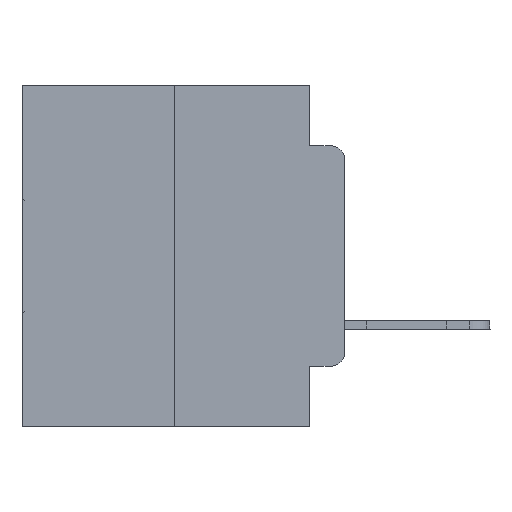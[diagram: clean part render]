
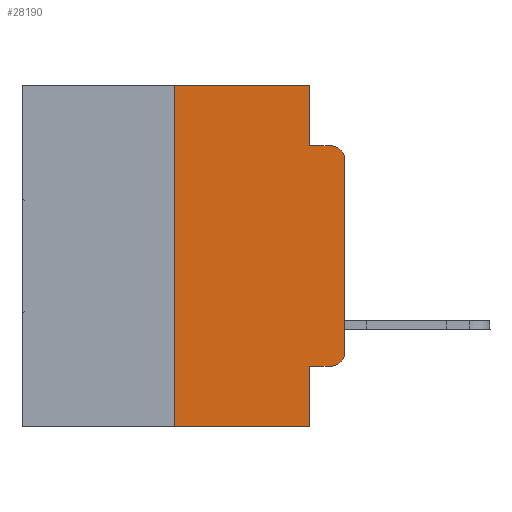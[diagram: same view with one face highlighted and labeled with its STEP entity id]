
A CAD part, left-side view. The second image highlights one B-rep face of the part: STEP entity #28190.
In plain terms, the highlighted planar face has unit normal (-1, 0, 0).
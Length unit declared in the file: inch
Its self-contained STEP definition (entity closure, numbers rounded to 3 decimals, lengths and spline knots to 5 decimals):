
#272 = ORIENTED_EDGE ( 'NONE', *, *, #9344, .T. ) ;
#401 = DIRECTION ( 'NONE',  ( 0., 0., 1. ) ) ;
#412 = DIRECTION ( 'NONE',  ( 0., -1., 0. ) ) ;
#505 = EDGE_CURVE ( 'NONE', #2118, #6179, #15809, .T. ) ;
#654 = DIRECTION ( 'NONE',  ( 0., 0., -1. ) ) ;
#1285 = CARTESIAN_POINT ( 'NONE',  ( 0., 0., -0.1085 ) ) ;
#1287 = EDGE_CURVE ( 'NONE', #6179, #3127, #4255, .T. ) ;
#1411 = ORIENTED_EDGE ( 'NONE', *, *, #1287, .F. ) ;
#1731 = ORIENTED_EDGE ( 'NONE', *, *, #11826, .T. ) ;
#1916 = CARTESIAN_POINT ( 'NONE',  ( 0., 0.051, -0.4115 ) ) ;
#2118 = VERTEX_POINT ( 'NONE', #9834 ) ;
#2252 = DIRECTION ( 'NONE',  ( 0., -1., 0. ) ) ;
#2348 = VECTOR ( 'NONE', #401, 39.37008 ) ;
#2408 = CARTESIAN_POINT ( 'NONE',  ( 0., 0.051, 0. ) ) ;
#2770 = ORIENTED_EDGE ( 'NONE', *, *, #24158, .T. ) ;
#2787 = ORIENTED_EDGE ( 'NONE', *, *, #505, .F. ) ;
#2824 = VECTOR ( 'NONE', #412, 39.37008 ) ;
#3104 = VECTOR ( 'NONE', #654, 39.37008 ) ;
#3127 = VERTEX_POINT ( 'NONE', #27790 ) ;
#3255 = AXIS2_PLACEMENT_3D ( 'NONE', #25083, #20595, #9284 ) ;
#4231 = EDGE_CURVE ( 'NONE', #3127, #21134, #23001, .T. ) ;
#4255 = LINE ( 'NONE', #17198, #11374 ) ;
#5452 = EDGE_CURVE ( 'NONE', #13313, #21204, #11567, .T. ) ;
#5498 = PLANE ( 'NONE',  #3255 ) ;
#5711 = ORIENTED_EDGE ( 'NONE', *, *, #4231, .F. ) ;
#5807 = DIRECTION ( 'NONE',  ( -1., 0., 0. ) ) ;
#6179 = VERTEX_POINT ( 'NONE', #23401 ) ;
#6425 = CIRCLE ( 'NONE', #8712, 0.02 ) ;
#6933 = EDGE_CURVE ( 'NONE', #21134, #28628, #18291, .T. ) ;
#7229 = DIRECTION ( 'NONE',  ( 0., 0., -1. ) ) ;
#7231 = EDGE_CURVE ( 'NONE', #9065, #22867, #11198, .T. ) ;
#7920 = ORIENTED_EDGE ( 'NONE', *, *, #5452, .F. ) ;
#7997 = VERTEX_POINT ( 'NONE', #19237 ) ;
#8314 = VECTOR ( 'NONE', #28692, 39.37008 ) ;
#8712 = AXIS2_PLACEMENT_3D ( 'NONE', #23764, #5807, #10313 ) ;
#8883 = AXIS2_PLACEMENT_3D ( 'NONE', #11729, #18106, #7229 ) ;
#8942 = CARTESIAN_POINT ( 'NONE',  ( 0., 0.473, -0.5 ) ) ;
#9042 = CARTESIAN_POINT ( 'NONE',  ( 0., 0.051, -0.5 ) ) ;
#9065 = VERTEX_POINT ( 'NONE', #23035 ) ;
#9284 = DIRECTION ( 'NONE',  ( 0., 0., -1. ) ) ;
#9344 = EDGE_CURVE ( 'NONE', #2118, #21204, #12870, .T. ) ;
#9834 = CARTESIAN_POINT ( 'NONE',  ( 0., 0.25, -0.5 ) ) ;
#9914 = ORIENTED_EDGE ( 'NONE', *, *, #6933, .F. ) ;
#10313 = DIRECTION ( 'NONE',  ( 0., 0., -1. ) ) ;
#10502 = LINE ( 'NONE', #1916, #19533 ) ;
#10763 = CARTESIAN_POINT ( 'NONE',  ( 0., 0., 0. ) ) ;
#11090 = EDGE_CURVE ( 'NONE', #22867, #28628, #26488, .T. ) ;
#11198 = LINE ( 'NONE', #10763, #23238 ) ;
#11374 = VECTOR ( 'NONE', #26472, 39.37008 ) ;
#11567 = LINE ( 'NONE', #2408, #8314 ) ;
#11615 = CARTESIAN_POINT ( 'NONE',  ( 0., 0.051, -0.0885 ) ) ;
#11729 = CARTESIAN_POINT ( 'NONE',  ( 0., 0.02, -0.1085 ) ) ;
#11826 = EDGE_CURVE ( 'NONE', #13313, #7997, #10502, .T. ) ;
#12515 = CARTESIAN_POINT ( 'NONE',  ( 0., 0.051, -0.4115 ) ) ;
#12870 = LINE ( 'NONE', #8942, #13627 ) ;
#13313 = VERTEX_POINT ( 'NONE', #12515 ) ;
#13627 = VECTOR ( 'NONE', #2252, 39.37008 ) ;
#15574 = CARTESIAN_POINT ( 'NONE',  ( 0., 0.051, -0.0885 ) ) ;
#15809 = LINE ( 'NONE', #27410, #2348 ) ;
#16065 = CARTESIAN_POINT ( 'NONE',  ( 0., 0.051, 0. ) ) ;
#17198 = CARTESIAN_POINT ( 'NONE',  ( 0., 0.473, 0. ) ) ;
#17286 = DIRECTION ( 'NONE',  ( 0., 0., 1. ) ) ;
#18106 = DIRECTION ( 'NONE',  ( -1., 0., 0. ) ) ;
#18291 = LINE ( 'NONE', #11615, #2824 ) ;
#19237 = CARTESIAN_POINT ( 'NONE',  ( 0., 0.02, -0.4115 ) ) ;
#19533 = VECTOR ( 'NONE', #28199, 39.37008 ) ;
#20595 = DIRECTION ( 'NONE',  ( 1., 0., 0. ) ) ;
#20657 = EDGE_LOOP ( 'NONE', ( #26353, #25692, #9914, #5711, #1411, #2787, #272, #7920, #1731, #2770 ) ) ;
#21134 = VERTEX_POINT ( 'NONE', #15574 ) ;
#21204 = VERTEX_POINT ( 'NONE', #9042 ) ;
#22867 = VERTEX_POINT ( 'NONE', #1285 ) ;
#22876 = CARTESIAN_POINT ( 'NONE',  ( 0., 0.02, -0.0885 ) ) ;
#23001 = LINE ( 'NONE', #16065, #3104 ) ;
#23035 = CARTESIAN_POINT ( 'NONE',  ( 0., 0., -0.3915 ) ) ;
#23238 = VECTOR ( 'NONE', #17286, 39.37008 ) ;
#23401 = CARTESIAN_POINT ( 'NONE',  ( 0., 0.25, 0. ) ) ;
#23764 = CARTESIAN_POINT ( 'NONE',  ( 0., 0.02, -0.3915 ) ) ;
#24158 = EDGE_CURVE ( 'NONE', #7997, #9065, #6425, .T. ) ;
#25083 = CARTESIAN_POINT ( 'NONE',  ( 0., 0.473, 0. ) ) ;
#25692 = ORIENTED_EDGE ( 'NONE', *, *, #11090, .T. ) ;
#26353 = ORIENTED_EDGE ( 'NONE', *, *, #7231, .T. ) ;
#26472 = DIRECTION ( 'NONE',  ( 0., -1., 0. ) ) ;
#26488 = CIRCLE ( 'NONE', #8883, 0.02 ) ;
#27273 = FACE_OUTER_BOUND ( 'NONE', #20657, .T. ) ;
#27410 = CARTESIAN_POINT ( 'NONE',  ( 0., 0.25, 0. ) ) ;
#27790 = CARTESIAN_POINT ( 'NONE',  ( 0., 0.051, 0. ) ) ;
#28190 = ADVANCED_FACE ( 'NONE', ( #27273 ), #5498, .F. ) ;
#28199 = DIRECTION ( 'NONE',  ( 0., -1., 0. ) ) ;
#28628 = VERTEX_POINT ( 'NONE', #22876 ) ;
#28692 = DIRECTION ( 'NONE',  ( 0., 0., -1. ) ) ;
